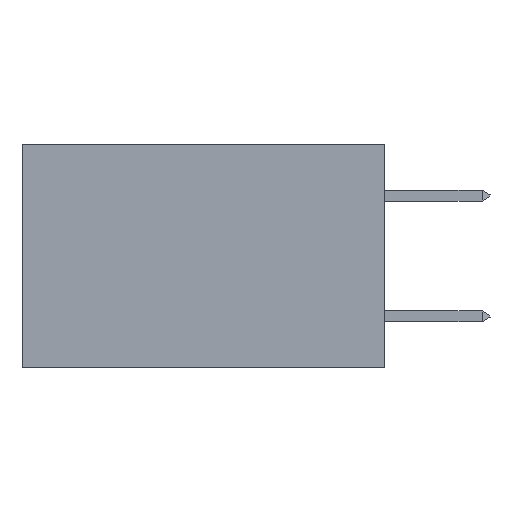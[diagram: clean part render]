
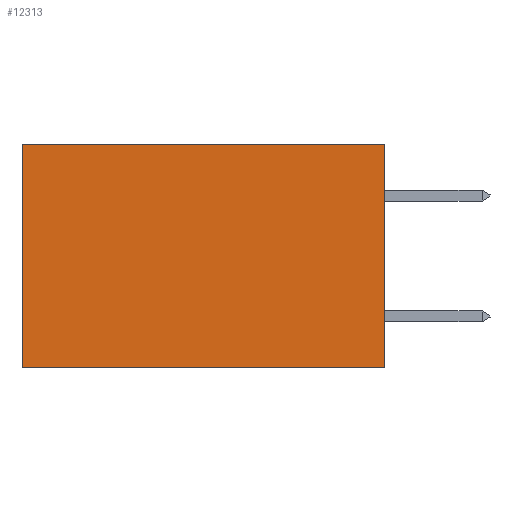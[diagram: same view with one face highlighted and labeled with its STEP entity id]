
A CAD part, left-side view. The second image highlights one B-rep face of the part: STEP entity #12313.
In plain terms, the highlighted planar face has unit normal (-1, 0, 0).
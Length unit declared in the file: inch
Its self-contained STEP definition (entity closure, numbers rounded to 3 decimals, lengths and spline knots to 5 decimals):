
#104 = EDGE_CURVE ( 'NONE', #6665, #11101, #4739, .T. ) ;
#1258 = CARTESIAN_POINT ( 'NONE',  ( 0.2875, 0., 0. ) ) ;
#2361 = CARTESIAN_POINT ( 'NONE',  ( 0.2875, 0.6, 0. ) ) ;
#2535 = DIRECTION ( 'NONE',  ( 0., 1., 0. ) ) ;
#3819 = PLANE ( 'NONE',  #25515 ) ;
#4069 = VECTOR ( 'NONE', #12437, 39.37008 ) ;
#4739 = LINE ( 'NONE', #8302, #4069 ) ;
#5750 = LINE ( 'NONE', #11266, #27410 ) ;
#6665 = VERTEX_POINT ( 'NONE', #1258 ) ;
#7970 = VECTOR ( 'NONE', #25641, 39.37008 ) ;
#8302 = CARTESIAN_POINT ( 'NONE',  ( 0.2875, 0., 0. ) ) ;
#8626 = FACE_OUTER_BOUND ( 'NONE', #14377, .T. ) ;
#10497 = VERTEX_POINT ( 'NONE', #27473 ) ;
#11101 = VERTEX_POINT ( 'NONE', #21404 ) ;
#11266 = CARTESIAN_POINT ( 'NONE',  ( 0.2875, 0., -0.37 ) ) ;
#12298 = CARTESIAN_POINT ( 'NONE',  ( 0.2875, 0., 0. ) ) ;
#12313 = ADVANCED_FACE ( 'NONE', ( #8626 ), #3819, .F. ) ;
#12437 = DIRECTION ( 'NONE',  ( 0., 0., -1. ) ) ;
#12525 = EDGE_CURVE ( 'NONE', #19675, #10497, #25962, .T. ) ;
#14377 = EDGE_LOOP ( 'NONE', ( #24209, #22758, #21261, #22426 ) ) ;
#14632 = DIRECTION ( 'NONE',  ( 0., 0., -1. ) ) ;
#18777 = CARTESIAN_POINT ( 'NONE',  ( 0.2875, 0.6, 0. ) ) ;
#19675 = VERTEX_POINT ( 'NONE', #18777 ) ;
#20645 = DIRECTION ( 'NONE',  ( 0., 1., 0. ) ) ;
#21261 = ORIENTED_EDGE ( 'NONE', *, *, #104, .F. ) ;
#21404 = CARTESIAN_POINT ( 'NONE',  ( 0.2875, 0., -0.37 ) ) ;
#21557 = LINE ( 'NONE', #12298, #22187 ) ;
#22187 = VECTOR ( 'NONE', #20645, 39.37008 ) ;
#22426 = ORIENTED_EDGE ( 'NONE', *, *, #27047, .T. ) ;
#22758 = ORIENTED_EDGE ( 'NONE', *, *, #24678, .F. ) ;
#22934 = CARTESIAN_POINT ( 'NONE',  ( 0.2875, 0., 0. ) ) ;
#24209 = ORIENTED_EDGE ( 'NONE', *, *, #12525, .T. ) ;
#24678 = EDGE_CURVE ( 'NONE', #11101, #10497, #5750, .T. ) ;
#25515 = AXIS2_PLACEMENT_3D ( 'NONE', #22934, #27011, #14632 ) ;
#25641 = DIRECTION ( 'NONE',  ( 0., 0., -1. ) ) ;
#25962 = LINE ( 'NONE', #2361, #7970 ) ;
#27011 = DIRECTION ( 'NONE',  ( 1., 0., 0. ) ) ;
#27047 = EDGE_CURVE ( 'NONE', #6665, #19675, #21557, .T. ) ;
#27410 = VECTOR ( 'NONE', #2535, 39.37008 ) ;
#27473 = CARTESIAN_POINT ( 'NONE',  ( 0.2875, 0.6, -0.37 ) ) ;
